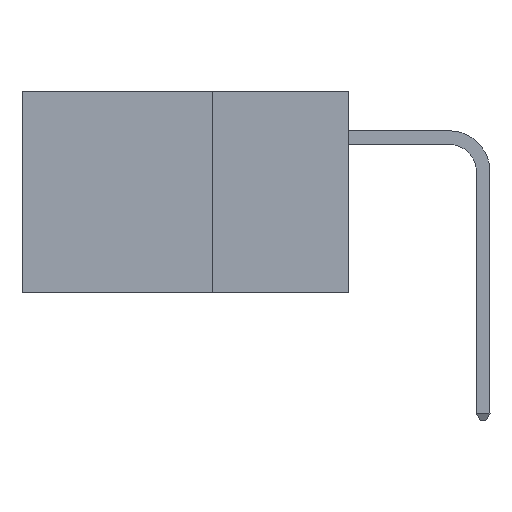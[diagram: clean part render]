
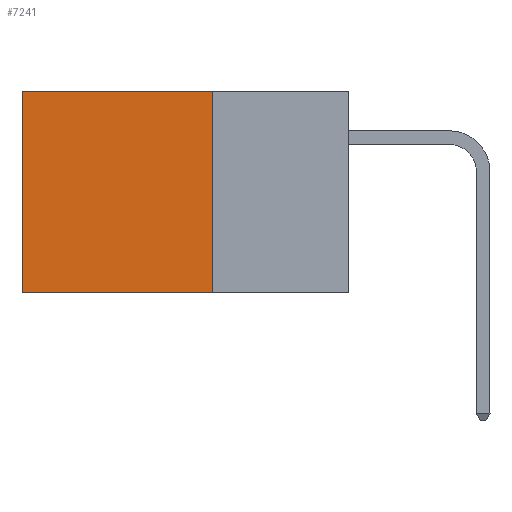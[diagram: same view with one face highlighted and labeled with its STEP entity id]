
A CAD part, left-side view. The second image highlights one B-rep face of the part: STEP entity #7241.
In plain terms, the highlighted planar face has unit normal (-1, 0, 0).
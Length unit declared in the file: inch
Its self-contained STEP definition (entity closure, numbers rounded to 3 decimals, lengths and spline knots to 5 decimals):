
#65 = PLANE ( 'NONE',  #8749 ) ;
#227 = DIRECTION ( 'NONE',  ( 0., 0., -1. ) ) ;
#643 = CARTESIAN_POINT ( 'NONE',  ( 0.2875, 0.6, 0. ) ) ;
#935 = CARTESIAN_POINT ( 'NONE',  ( 0.2875, 0.25, 0. ) ) ;
#1113 = CARTESIAN_POINT ( 'NONE',  ( 0.2875, 0.25, 0. ) ) ;
#1493 = EDGE_LOOP ( 'NONE', ( #8856, #8319, #7875, #5108 ) ) ;
#1496 = LINE ( 'NONE', #4237, #5962 ) ;
#1718 = LINE ( 'NONE', #11627, #3729 ) ;
#1848 = VERTEX_POINT ( 'NONE', #643 ) ;
#2192 = VERTEX_POINT ( 'NONE', #1113 ) ;
#3067 = DIRECTION ( 'NONE',  ( 0., 1., 0. ) ) ;
#3655 = DIRECTION ( 'NONE',  ( 1., 0., 0. ) ) ;
#3729 = VECTOR ( 'NONE', #9027, 39.37008 ) ;
#4237 = CARTESIAN_POINT ( 'NONE',  ( 0.2875, 0.25, -0.37 ) ) ;
#4476 = FACE_OUTER_BOUND ( 'NONE', #1493, .T. ) ;
#4542 = EDGE_CURVE ( 'NONE', #1848, #9610, #1718, .T. ) ;
#5108 = ORIENTED_EDGE ( 'NONE', *, *, #5745, .T. ) ;
#5745 = EDGE_CURVE ( 'NONE', #2192, #1848, #11281, .T. ) ;
#5834 = CARTESIAN_POINT ( 'NONE',  ( 0.2875, 0.25, 0. ) ) ;
#5959 = EDGE_CURVE ( 'NONE', #10930, #9610, #1496, .T. ) ;
#5962 = VECTOR ( 'NONE', #8220, 39.37008 ) ;
#6258 = VECTOR ( 'NONE', #227, 39.37008 ) ;
#6926 = VECTOR ( 'NONE', #3067, 39.37008 ) ;
#7241 = ADVANCED_FACE ( 'NONE', ( #4476 ), #65, .F. ) ;
#7875 = ORIENTED_EDGE ( 'NONE', *, *, #10605, .F. ) ;
#8166 = DIRECTION ( 'NONE',  ( 0., 0., -1. ) ) ;
#8220 = DIRECTION ( 'NONE',  ( 0., 1., 0. ) ) ;
#8319 = ORIENTED_EDGE ( 'NONE', *, *, #5959, .F. ) ;
#8749 = AXIS2_PLACEMENT_3D ( 'NONE', #9984, #3655, #8166 ) ;
#8856 = ORIENTED_EDGE ( 'NONE', *, *, #4542, .T. ) ;
#8875 = CARTESIAN_POINT ( 'NONE',  ( 0.2875, 0.25, -0.37 ) ) ;
#9027 = DIRECTION ( 'NONE',  ( 0., 0., -1. ) ) ;
#9610 = VERTEX_POINT ( 'NONE', #10758 ) ;
#9984 = CARTESIAN_POINT ( 'NONE',  ( 0.2875, 0.25, 0. ) ) ;
#10605 = EDGE_CURVE ( 'NONE', #2192, #10930, #10788, .T. ) ;
#10758 = CARTESIAN_POINT ( 'NONE',  ( 0.2875, 0.6, -0.37 ) ) ;
#10788 = LINE ( 'NONE', #935, #6258 ) ;
#10930 = VERTEX_POINT ( 'NONE', #8875 ) ;
#11281 = LINE ( 'NONE', #5834, #6926 ) ;
#11627 = CARTESIAN_POINT ( 'NONE',  ( 0.2875, 0.6, 0. ) ) ;
